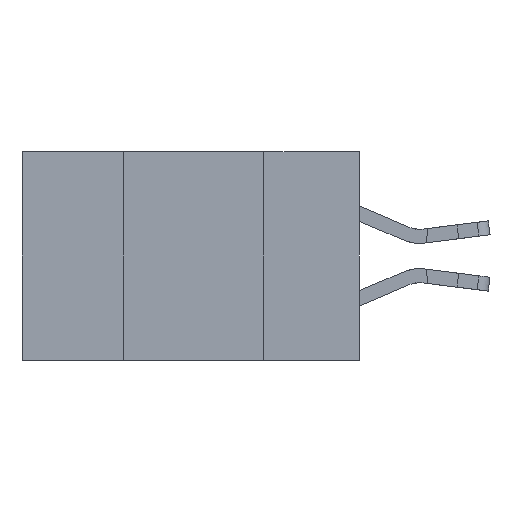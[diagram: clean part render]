
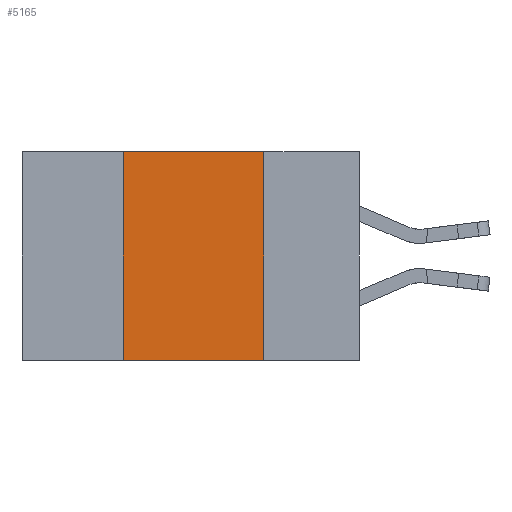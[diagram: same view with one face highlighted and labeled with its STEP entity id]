
A CAD part, left-side view. The second image highlights one B-rep face of the part: STEP entity #5165.
In plain terms, the highlighted planar face has unit normal (-1, 0, 0).
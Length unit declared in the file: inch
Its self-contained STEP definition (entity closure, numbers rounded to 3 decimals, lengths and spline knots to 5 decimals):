
#864 = DIRECTION ( 'NONE',  ( 0., 0., 1. ) ) ;
#1121 = CARTESIAN_POINT ( 'NONE',  ( 0., 0.6, -0.37 ) ) ;
#1125 = DIRECTION ( 'NONE',  ( 0., -1., 0. ) ) ;
#1431 = VECTOR ( 'NONE', #11092, 39.37008 ) ;
#1784 = PLANE ( 'NONE',  #12844 ) ;
#2841 = VECTOR ( 'NONE', #3196, 39.37008 ) ;
#3196 = DIRECTION ( 'NONE',  ( 0., 0., -1. ) ) ;
#3219 = EDGE_CURVE ( 'NONE', #15234, #6808, #14470, .T. ) ;
#3552 = DIRECTION ( 'NONE',  ( 1., 0., 0. ) ) ;
#4312 = FACE_OUTER_BOUND ( 'NONE', #8302, .T. ) ;
#5165 = ADVANCED_FACE ( 'NONE', ( #4312 ), #1784, .F. ) ;
#6077 = VECTOR ( 'NONE', #1125, 39.37008 ) ;
#6808 = VERTEX_POINT ( 'NONE', #15574 ) ;
#7121 = EDGE_CURVE ( 'NONE', #10581, #20133, #16015, .T. ) ;
#7198 = CARTESIAN_POINT ( 'NONE',  ( 0., 0.42, 0. ) ) ;
#7572 = ORIENTED_EDGE ( 'NONE', *, *, #7121, .F. ) ;
#8087 = ORIENTED_EDGE ( 'NONE', *, *, #20737, .F. ) ;
#8119 = CARTESIAN_POINT ( 'NONE',  ( 0., 0.17, 0. ) ) ;
#8302 = EDGE_LOOP ( 'NONE', ( #19664, #7572, #8087, #12832 ) ) ;
#10581 = VERTEX_POINT ( 'NONE', #7198 ) ;
#11028 = CARTESIAN_POINT ( 'NONE',  ( 0., 0.17, 0. ) ) ;
#11092 = DIRECTION ( 'NONE',  ( 0., -1., 0. ) ) ;
#11756 = LINE ( 'NONE', #20203, #19581 ) ;
#12832 = ORIENTED_EDGE ( 'NONE', *, *, #3219, .T. ) ;
#12844 = AXIS2_PLACEMENT_3D ( 'NONE', #19459, #3552, #14808 ) ;
#14470 = LINE ( 'NONE', #1121, #1431 ) ;
#14808 = DIRECTION ( 'NONE',  ( 0., 0., -1. ) ) ;
#15222 = LINE ( 'NONE', #8119, #2841 ) ;
#15234 = VERTEX_POINT ( 'NONE', #16300 ) ;
#15574 = CARTESIAN_POINT ( 'NONE',  ( 0., 0.17, -0.37 ) ) ;
#15876 = CARTESIAN_POINT ( 'NONE',  ( 0., 0.6, 0. ) ) ;
#16015 = LINE ( 'NONE', #15876, #6077 ) ;
#16300 = CARTESIAN_POINT ( 'NONE',  ( 0., 0.42, -0.37 ) ) ;
#18640 = EDGE_CURVE ( 'NONE', #20133, #6808, #15222, .T. ) ;
#19459 = CARTESIAN_POINT ( 'NONE',  ( 0., 0.6, 0. ) ) ;
#19581 = VECTOR ( 'NONE', #864, 39.37008 ) ;
#19664 = ORIENTED_EDGE ( 'NONE', *, *, #18640, .F. ) ;
#20133 = VERTEX_POINT ( 'NONE', #11028 ) ;
#20203 = CARTESIAN_POINT ( 'NONE',  ( 0., 0.42, 0. ) ) ;
#20737 = EDGE_CURVE ( 'NONE', #15234, #10581, #11756, .T. ) ;
